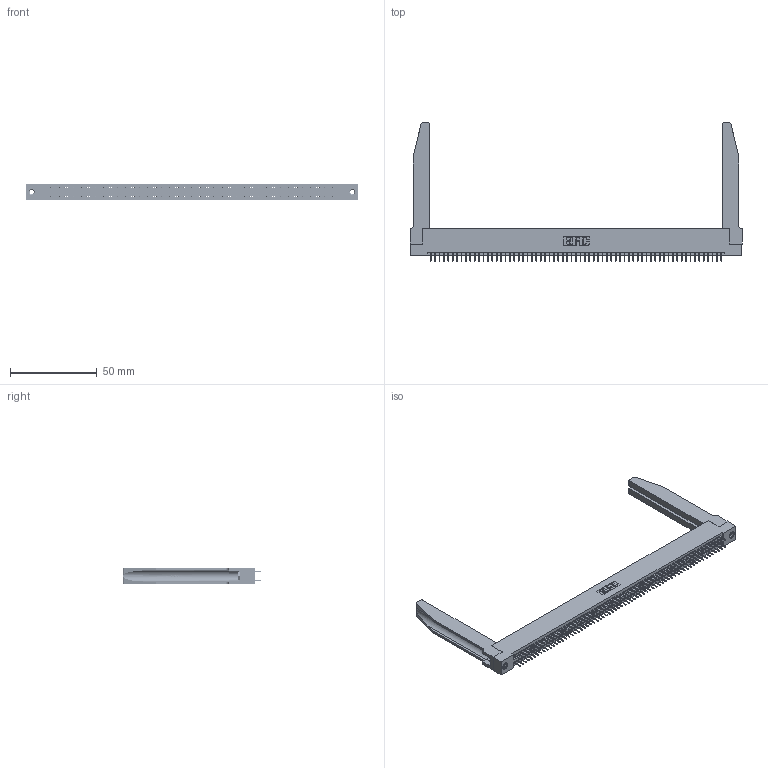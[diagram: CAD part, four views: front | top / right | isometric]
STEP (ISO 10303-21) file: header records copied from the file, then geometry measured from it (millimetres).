
FILE_DESCRIPTION (( 'STEP AP203' ), '1' );
FILE_NAME ('345-134-525-278.STEP', '2020-09-22T15:13:52', ( '' ), ( '' ), 'SwSTEP 2.0', 'SolidWorks 2020', '' );
FILE_SCHEMA (( 'CONFIG_CONTROL_DESIGN' ));
Length unit declared in the file: inch
Products named in the file (5): 345-292-001_345-293-125; 345-134-525-278; 345 Part_Flush Mounting Lugs - 0.156 Dia-TH; 345-250-001_345-250-001-102; 345-220-078_345-220-078
Assembly tree (139 placements, depth 2):
  345-134-525-278
    345 Part_Flush Mounting Lugs - 0.156 Dia-TH
    345-292-001_345-293-125  x134
    345-250-001_345-250-001-102  x2
    345-220-078_345-220-078  x2
Bounding box: 191.41 x 79.68 x 9.4 mm (x, y, z)
Volume: 26376.1 mm3; surface area: 34160.3 mm2
Topology: 139 solids, 139 shells, 7596 faces, 21451 edges, 13754 vertices
Faces by surface type: plane 5448, cylinder 2096, bspline 36, cone 12, torus 4
Entity records: 54018 total; most frequent: CARTESIAN_POINT 9947, ORIENTED_EDGE 8778, DIRECTION 7735, EDGE_CURVE 4389, LINE 3899, VECTOR 3899, VERTEX_POINT 2916, AXIS2_PLACEMENT_3D 1918
